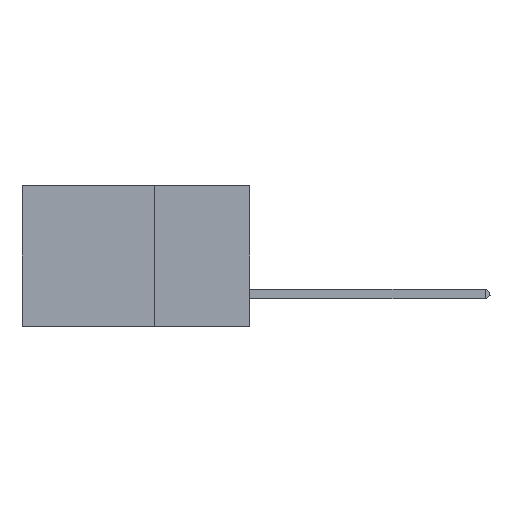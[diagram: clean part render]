
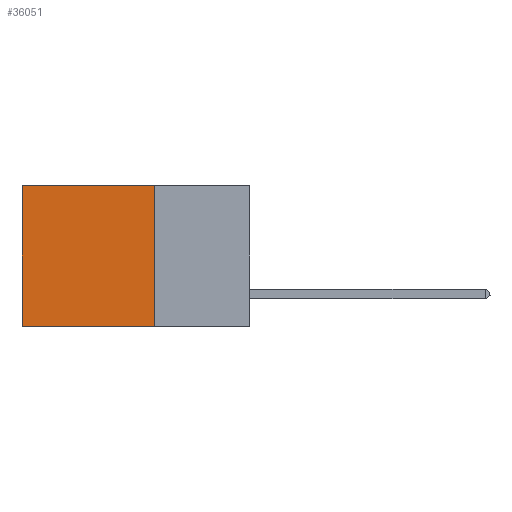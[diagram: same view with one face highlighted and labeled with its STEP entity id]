
A CAD part, left-side view. The second image highlights one B-rep face of the part: STEP entity #36051.
In plain terms, the highlighted planar face has unit normal (-1, 0, 0).
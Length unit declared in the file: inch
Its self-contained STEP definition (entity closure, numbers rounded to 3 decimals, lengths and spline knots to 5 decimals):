
#1356 = CARTESIAN_POINT ( 'NONE',  ( 0.2875, 0.25, 0. ) ) ;
#2211 = DIRECTION ( 'NONE',  ( 0., 0., -1. ) ) ;
#4703 = EDGE_CURVE ( 'NONE', #26357, #21985, #25469, .T. ) ;
#5935 = EDGE_LOOP ( 'NONE', ( #14024, #12920, #21194, #37823 ) ) ;
#7858 = DIRECTION ( 'NONE',  ( 0., 0., -1. ) ) ;
#9105 = DIRECTION ( 'NONE',  ( 1., 0., 0. ) ) ;
#11474 = CARTESIAN_POINT ( 'NONE',  ( 0.2875, 0.6, -0.37 ) ) ;
#12745 = DIRECTION ( 'NONE',  ( 0., 0., -1. ) ) ;
#12920 = ORIENTED_EDGE ( 'NONE', *, *, #15190, .F. ) ;
#13145 = FACE_OUTER_BOUND ( 'NONE', #5935, .T. ) ;
#14024 = ORIENTED_EDGE ( 'NONE', *, *, #4703, .T. ) ;
#15039 = VECTOR ( 'NONE', #7858, 39.37008 ) ;
#15190 = EDGE_CURVE ( 'NONE', #40329, #21985, #39576, .T. ) ;
#15896 = LINE ( 'NONE', #1356, #17050 ) ;
#16521 = VECTOR ( 'NONE', #23264, 39.37008 ) ;
#16800 = DIRECTION ( 'NONE',  ( 0., 1., 0. ) ) ;
#17050 = VECTOR ( 'NONE', #12745, 39.37008 ) ;
#21194 = ORIENTED_EDGE ( 'NONE', *, *, #37145, .F. ) ;
#21985 = VERTEX_POINT ( 'NONE', #11474 ) ;
#22805 = EDGE_CURVE ( 'NONE', #32586, #26357, #39657, .T. ) ;
#23264 = DIRECTION ( 'NONE',  ( 0., 1., 0. ) ) ;
#23826 = CARTESIAN_POINT ( 'NONE',  ( 0.2875, 0.25, 0. ) ) ;
#25469 = LINE ( 'NONE', #41278, #15039 ) ;
#26357 = VERTEX_POINT ( 'NONE', #28840 ) ;
#27128 = AXIS2_PLACEMENT_3D ( 'NONE', #23826, #9105, #2211 ) ;
#27486 = CARTESIAN_POINT ( 'NONE',  ( 0.2875, 0.25, 0. ) ) ;
#28617 = VECTOR ( 'NONE', #16800, 39.37008 ) ;
#28840 = CARTESIAN_POINT ( 'NONE',  ( 0.2875, 0.6, 0. ) ) ;
#32586 = VERTEX_POINT ( 'NONE', #45402 ) ;
#36051 = ADVANCED_FACE ( 'NONE', ( #13145 ), #46398, .F. ) ;
#37145 = EDGE_CURVE ( 'NONE', #32586, #40329, #15896, .T. ) ;
#37823 = ORIENTED_EDGE ( 'NONE', *, *, #22805, .T. ) ;
#38319 = CARTESIAN_POINT ( 'NONE',  ( 0.2875, 0.25, -0.37 ) ) ;
#39194 = CARTESIAN_POINT ( 'NONE',  ( 0.2875, 0.25, -0.37 ) ) ;
#39576 = LINE ( 'NONE', #38319, #28617 ) ;
#39657 = LINE ( 'NONE', #27486, #16521 ) ;
#40329 = VERTEX_POINT ( 'NONE', #39194 ) ;
#41278 = CARTESIAN_POINT ( 'NONE',  ( 0.2875, 0.6, 0. ) ) ;
#45402 = CARTESIAN_POINT ( 'NONE',  ( 0.2875, 0.25, 0. ) ) ;
#46398 = PLANE ( 'NONE',  #27128 ) ;
